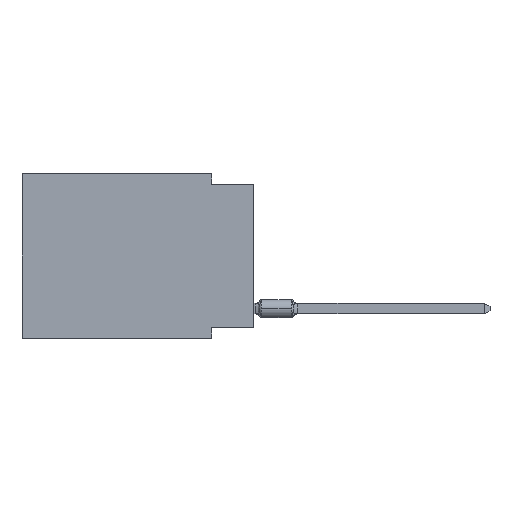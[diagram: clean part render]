
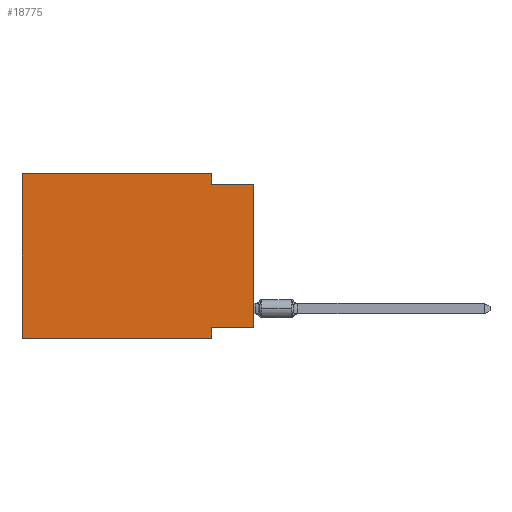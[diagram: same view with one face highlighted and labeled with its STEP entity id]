
A CAD part, left-side view. The second image highlights one B-rep face of the part: STEP entity #18775.
In plain terms, the highlighted planar face has unit normal (-1, 0, 0).
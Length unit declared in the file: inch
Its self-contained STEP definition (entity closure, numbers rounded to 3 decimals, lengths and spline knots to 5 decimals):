
#127 = EDGE_CURVE ( 'NONE', #2429, #9996, #5819, .T. ) ;
#135 = DIRECTION ( 'NONE',  ( 0., 0., -1. ) ) ;
#609 = LINE ( 'NONE', #14509, #9987 ) ;
#665 = VERTEX_POINT ( 'NONE', #15337 ) ;
#902 = DIRECTION ( 'NONE',  ( 0., 1., 0. ) ) ;
#942 = DIRECTION ( 'NONE',  ( 0., -1., 0. ) ) ;
#1489 = ORIENTED_EDGE ( 'NONE', *, *, #2580, .F. ) ;
#1908 = CARTESIAN_POINT ( 'NONE',  ( 0., 0.55, 0. ) ) ;
#1915 = DIRECTION ( 'NONE',  ( 0., 0., 1. ) ) ;
#2429 = VERTEX_POINT ( 'NONE', #2861 ) ;
#2452 = CARTESIAN_POINT ( 'NONE',  ( 0., 0.1, -0.365 ) ) ;
#2580 = EDGE_CURVE ( 'NONE', #10084, #12598, #2663, .T. ) ;
#2663 = LINE ( 'NONE', #8711, #9874 ) ;
#2840 = LINE ( 'NONE', #18044, #5339 ) ;
#2861 = CARTESIAN_POINT ( 'NONE',  ( 0., 0.1, -0.025 ) ) ;
#3301 = PLANE ( 'NONE',  #10942 ) ;
#3308 = LINE ( 'NONE', #10752, #12934 ) ;
#3362 = CARTESIAN_POINT ( 'NONE',  ( 0., 0., -0.025 ) ) ;
#3397 = FACE_OUTER_BOUND ( 'NONE', #16839, .T. ) ;
#4173 = EDGE_CURVE ( 'NONE', #19558, #12598, #2840, .T. ) ;
#4462 = ORIENTED_EDGE ( 'NONE', *, *, #9565, .F. ) ;
#5253 = ORIENTED_EDGE ( 'NONE', *, *, #7081, .F. ) ;
#5339 = VECTOR ( 'NONE', #5918, 39.37008 ) ;
#5609 = CARTESIAN_POINT ( 'NONE',  ( 0., 0.55, 0. ) ) ;
#5812 = LINE ( 'NONE', #10558, #19263 ) ;
#5819 = LINE ( 'NONE', #17848, #18055 ) ;
#5918 = DIRECTION ( 'NONE',  ( 0., -1., 0. ) ) ;
#6765 = CARTESIAN_POINT ( 'NONE',  ( 0., 0., 0. ) ) ;
#7081 = EDGE_CURVE ( 'NONE', #19558, #18859, #3308, .T. ) ;
#7196 = DIRECTION ( 'NONE',  ( 0., -1., 0. ) ) ;
#7578 = ORIENTED_EDGE ( 'NONE', *, *, #10597, .F. ) ;
#7992 = VECTOR ( 'NONE', #14029, 39.37008 ) ;
#8711 = CARTESIAN_POINT ( 'NONE',  ( 0., 0.1, -0.39 ) ) ;
#9412 = VERTEX_POINT ( 'NONE', #15462 ) ;
#9537 = VECTOR ( 'NONE', #942, 39.37008 ) ;
#9565 = EDGE_CURVE ( 'NONE', #18859, #665, #15665, .T. ) ;
#9874 = VECTOR ( 'NONE', #14788, 39.37008 ) ;
#9987 = VECTOR ( 'NONE', #902, 39.37008 ) ;
#9996 = VERTEX_POINT ( 'NONE', #3362 ) ;
#10084 = VERTEX_POINT ( 'NONE', #2452 ) ;
#10558 = CARTESIAN_POINT ( 'NONE',  ( 0., 0.1, 0. ) ) ;
#10597 = EDGE_CURVE ( 'NONE', #665, #2429, #5812, .T. ) ;
#10744 = CARTESIAN_POINT ( 'NONE',  ( 0., 0.55, 0. ) ) ;
#10752 = CARTESIAN_POINT ( 'NONE',  ( 0., 0.55, 0. ) ) ;
#10942 = AXIS2_PLACEMENT_3D ( 'NONE', #1908, #15424, #13922 ) ;
#11236 = LINE ( 'NONE', #6765, #7992 ) ;
#11982 = ORIENTED_EDGE ( 'NONE', *, *, #16997, .T. ) ;
#12534 = ORIENTED_EDGE ( 'NONE', *, *, #127, .F. ) ;
#12598 = VERTEX_POINT ( 'NONE', #18189 ) ;
#12934 = VECTOR ( 'NONE', #1915, 39.37008 ) ;
#13922 = DIRECTION ( 'NONE',  ( 0., 0., -1. ) ) ;
#14029 = DIRECTION ( 'NONE',  ( 0., 0., 1. ) ) ;
#14509 = CARTESIAN_POINT ( 'NONE',  ( 0., 0., -0.365 ) ) ;
#14788 = DIRECTION ( 'NONE',  ( 0., 0., -1. ) ) ;
#15337 = CARTESIAN_POINT ( 'NONE',  ( 0., 0.1, 0. ) ) ;
#15424 = DIRECTION ( 'NONE',  ( 1., 0., 0. ) ) ;
#15462 = CARTESIAN_POINT ( 'NONE',  ( 0., 0., -0.365 ) ) ;
#15665 = LINE ( 'NONE', #5609, #9537 ) ;
#16839 = EDGE_LOOP ( 'NONE', ( #11982, #12534, #7578, #4462, #5253, #18567, #1489, #17208 ) ) ;
#16997 = EDGE_CURVE ( 'NONE', #9412, #9996, #11236, .T. ) ;
#17208 = ORIENTED_EDGE ( 'NONE', *, *, #18978, .F. ) ;
#17848 = CARTESIAN_POINT ( 'NONE',  ( 0., 0., -0.025 ) ) ;
#18044 = CARTESIAN_POINT ( 'NONE',  ( 0., 0.55, -0.39 ) ) ;
#18055 = VECTOR ( 'NONE', #7196, 39.37008 ) ;
#18189 = CARTESIAN_POINT ( 'NONE',  ( 0., 0.1, -0.39 ) ) ;
#18567 = ORIENTED_EDGE ( 'NONE', *, *, #4173, .T. ) ;
#18775 = ADVANCED_FACE ( 'NONE', ( #3397 ), #3301, .F. ) ;
#18859 = VERTEX_POINT ( 'NONE', #10744 ) ;
#18978 = EDGE_CURVE ( 'NONE', #9412, #10084, #609, .T. ) ;
#19263 = VECTOR ( 'NONE', #135, 39.37008 ) ;
#19451 = CARTESIAN_POINT ( 'NONE',  ( 0., 0.55, -0.39 ) ) ;
#19558 = VERTEX_POINT ( 'NONE', #19451 ) ;
